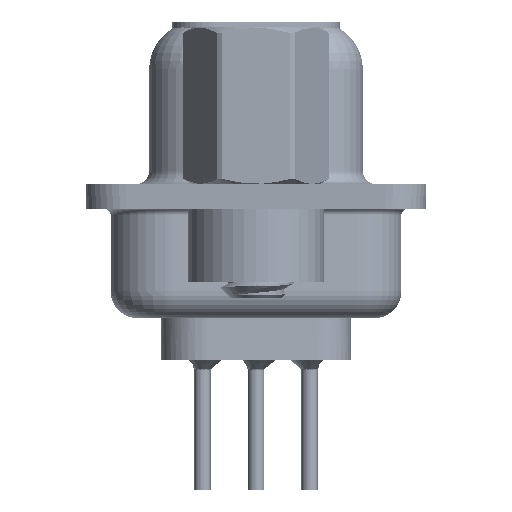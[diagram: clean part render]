
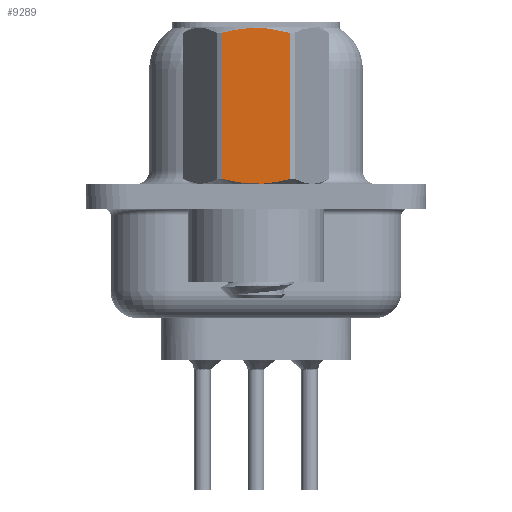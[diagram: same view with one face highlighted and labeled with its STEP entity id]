
A CAD part, left-side view. The second image highlights one B-rep face of the part: STEP entity #9289.
In plain terms, the highlighted planar face has unit normal (-1, 0, 0).
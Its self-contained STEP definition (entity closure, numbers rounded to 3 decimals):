
#759 = CARTESIAN_POINT ( 'NONE',  ( -2.381, 0.853, 6.151 ) ) ;
#2321 = VECTOR ( 'NONE', #33473, 1000. ) ;
#3811 = CARTESIAN_POINT ( 'NONE',  ( -2.381, -1.273, 6.048 ) ) ;
#3999 = CARTESIAN_POINT ( 'NONE',  ( -2.381, -0.215, 6.232 ) ) ;
#4881 = VERTEX_POINT ( 'NONE', #32948 ) ;
#5337 = CARTESIAN_POINT ( 'NONE',  ( -2.381, -0.858, 0.55 ) ) ;
#5597 = B_SPLINE_CURVE_WITH_KNOTS ( 'NONE', 3,
 ( #17138, #17327, #10903, #22490, #22850, #34129, #16957, #5337, #8587, #34309 ),
 .UNSPECIFIED., .F., .F.,
 ( 4, 2, 2, 2, 4 ),
 ( 0.003, 0.003, 0.004, 0.004, 0.005 ),
 .UNSPECIFIED. ) ;
#5792 = DIRECTION ( 'NONE',  ( -1., 0., 0. ) ) ;
#5983 = PLANE ( 'NONE',  #28200 ) ;
#6056 = EDGE_CURVE ( 'NONE', #31754, #4881, #17459, .T. ) ;
#6477 = CARTESIAN_POINT ( 'NONE',  ( -2.381, 1.273, 6.048 ) ) ;
#6866 = CARTESIAN_POINT ( 'NONE',  ( -2.381, -0.858, 6.15 ) ) ;
#7712 = EDGE_CURVE ( 'NONE', #32061, #29328, #21837, .T. ) ;
#8587 = CARTESIAN_POINT ( 'NONE',  ( -2.381, -1.066, 0.596 ) ) ;
#9289 = ADVANCED_FACE ( 'NONE', ( #34575 ), #5983, .T. ) ;
#9353 = CARTESIAN_POINT ( 'NONE',  ( -2.381, -0.432, 6.215 ) ) ;
#10575 = VECTOR ( 'NONE', #23173, 1000. ) ;
#10596 = EDGE_CURVE ( 'NONE', #4881, #32061, #21518, .T. ) ;
#10903 = CARTESIAN_POINT ( 'NONE',  ( -2.381, 0.853, 0.549 ) ) ;
#11904 = EDGE_LOOP ( 'NONE', ( #34934, #35556, #37554, #36263 ) ) ;
#14575 = DIRECTION ( 'NONE',  ( 0., -1., 0. ) ) ;
#16957 = CARTESIAN_POINT ( 'NONE',  ( -2.381, -0.432, 0.485 ) ) ;
#17138 = CARTESIAN_POINT ( 'NONE',  ( -2.381, 1.273, 0.652 ) ) ;
#17327 = CARTESIAN_POINT ( 'NONE',  ( -2.381, 1.065, 0.596 ) ) ;
#17459 = LINE ( 'NONE', #34079, #10575 ) ;
#17901 = CARTESIAN_POINT ( 'NONE',  ( -2.381, 0.215, 6.232 ) ) ;
#19349 = CARTESIAN_POINT ( 'NONE',  ( -2.381, 1.273, 3.792 ) ) ;
#20948 = CARTESIAN_POINT ( 'NONE',  ( -2.381, 0.428, 6.215 ) ) ;
#21518 = B_SPLINE_CURVE_WITH_KNOTS ( 'NONE', 3,
 ( #3811, #35447, #6866, #9353, #3999, #17901, #20948, #759, #32590, #6477 ),
 .UNSPECIFIED., .F., .F.,
 ( 4, 2, 2, 2, 4 ),
 ( 0.001, 0.002, 0.002, 0.003, 0.004 ),
 .UNSPECIFIED. ) ;
#21837 = LINE ( 'NONE', #19349, #2321 ) ;
#22490 = CARTESIAN_POINT ( 'NONE',  ( -2.381, 0.428, 0.485 ) ) ;
#22850 = CARTESIAN_POINT ( 'NONE',  ( -2.381, 0.215, 0.468 ) ) ;
#23173 = DIRECTION ( 'NONE',  ( 0., 0., 1. ) ) ;
#24913 = CARTESIAN_POINT ( 'NONE',  ( -2.381, 1.273, 0.652 ) ) ;
#26525 = CARTESIAN_POINT ( 'NONE',  ( -2.381, 1.273, 6.048 ) ) ;
#28200 = AXIS2_PLACEMENT_3D ( 'NONE', #29033, #5792, #14575 ) ;
#29033 = CARTESIAN_POINT ( 'NONE',  ( -2.381, 1.375, -3.75 ) ) ;
#29195 = CARTESIAN_POINT ( 'NONE',  ( -2.381, -1.273, 0.652 ) ) ;
#29328 = VERTEX_POINT ( 'NONE', #24913 ) ;
#31498 = EDGE_CURVE ( 'NONE', #29328, #31754, #5597, .T. ) ;
#31754 = VERTEX_POINT ( 'NONE', #29195 ) ;
#32061 = VERTEX_POINT ( 'NONE', #26525 ) ;
#32590 = CARTESIAN_POINT ( 'NONE',  ( -2.381, 1.065, 6.104 ) ) ;
#32948 = CARTESIAN_POINT ( 'NONE',  ( -2.381, -1.273, 6.048 ) ) ;
#33473 = DIRECTION ( 'NONE',  ( 0., 0., -1. ) ) ;
#34079 = CARTESIAN_POINT ( 'NONE',  ( -2.381, -1.273, 3.792 ) ) ;
#34129 = CARTESIAN_POINT ( 'NONE',  ( -2.381, -0.215, 0.468 ) ) ;
#34309 = CARTESIAN_POINT ( 'NONE',  ( -2.381, -1.273, 0.652 ) ) ;
#34575 = FACE_OUTER_BOUND ( 'NONE', #11904, .T. ) ;
#34934 = ORIENTED_EDGE ( 'NONE', *, *, #31498, .T. ) ;
#35447 = CARTESIAN_POINT ( 'NONE',  ( -2.381, -1.066, 6.104 ) ) ;
#35556 = ORIENTED_EDGE ( 'NONE', *, *, #6056, .T. ) ;
#36263 = ORIENTED_EDGE ( 'NONE', *, *, #7712, .T. ) ;
#37554 = ORIENTED_EDGE ( 'NONE', *, *, #10596, .T. ) ;
